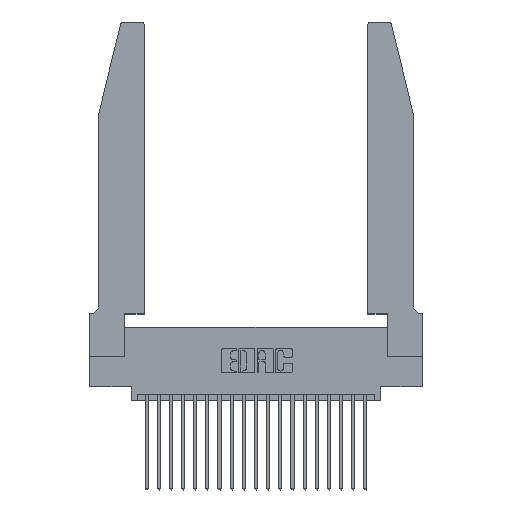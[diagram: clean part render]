
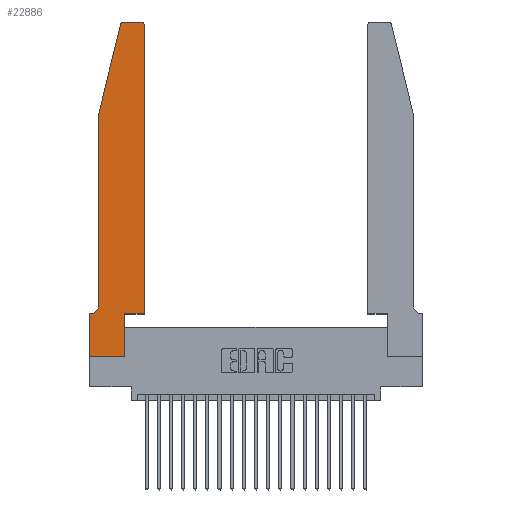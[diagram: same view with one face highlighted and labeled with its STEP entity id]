
A CAD part, top view. The second image highlights one B-rep face of the part: STEP entity #22886.
In plain terms, the highlighted planar face has unit normal (0, 0, 1).
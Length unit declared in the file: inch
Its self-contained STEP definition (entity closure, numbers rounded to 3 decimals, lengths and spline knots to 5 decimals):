
#38 = CIRCLE ( 'NONE', #16326, 0.07 ) ;
#225 = DIRECTION ( 'NONE',  ( 0., -1., 0. ) ) ;
#244 = VERTEX_POINT ( 'NONE', #14254 ) ;
#664 = VECTOR ( 'NONE', #12266, 39.37008 ) ;
#784 = DIRECTION ( 'NONE',  ( -1., 0., 0. ) ) ;
#834 = ORIENTED_EDGE ( 'NONE', *, *, #2104, .T. ) ;
#944 = ORIENTED_EDGE ( 'NONE', *, *, #11336, .T. ) ;
#1945 = ORIENTED_EDGE ( 'NONE', *, *, #15165, .T. ) ;
#2104 = EDGE_CURVE ( 'NONE', #244, #15278, #16944, .T. ) ;
#2153 = DIRECTION ( 'NONE',  ( 0., 0., 1. ) ) ;
#2366 = VERTEX_POINT ( 'NONE', #15646 ) ;
#2479 = EDGE_CURVE ( 'NONE', #20971, #8967, #14375, .T. ) ;
#3128 = AXIS2_PLACEMENT_3D ( 'NONE', #17118, #6433, #18855 ) ;
#3264 = DIRECTION ( 'NONE',  ( 1., 0., 0. ) ) ;
#3488 = DIRECTION ( 'NONE',  ( -1., 0., 0. ) ) ;
#3572 = ORIENTED_EDGE ( 'NONE', *, *, #12451, .T. ) ;
#3881 = PLANE ( 'NONE',  #18266 ) ;
#4040 = LINE ( 'NONE', #9130, #7724 ) ;
#4119 = VERTEX_POINT ( 'NONE', #5411 ) ;
#4292 = VECTOR ( 'NONE', #3488, 39.37008 ) ;
#4892 = DIRECTION ( 'NONE',  ( 0., 0., 1. ) ) ;
#4905 = LINE ( 'NONE', #13172, #14984 ) ;
#5411 = CARTESIAN_POINT ( 'NONE',  ( 0.0755, 2., 0.37 ) ) ;
#5440 = LINE ( 'NONE', #19428, #4292 ) ;
#6240 = CARTESIAN_POINT ( 'NONE',  ( 0.4505, 0.35, 0.37 ) ) ;
#6275 = FACE_OUTER_BOUND ( 'NONE', #11863, .T. ) ;
#6433 = DIRECTION ( 'NONE',  ( 0., 0., 1. ) ) ;
#6575 = ORIENTED_EDGE ( 'NONE', *, *, #20298, .T. ) ;
#6600 = VECTOR ( 'NONE', #225, 39.37008 ) ;
#6689 = ORIENTED_EDGE ( 'NONE', *, *, #2479, .T. ) ;
#7184 = VECTOR ( 'NONE', #18664, 39.37008 ) ;
#7588 = CARTESIAN_POINT ( 'NONE',  ( 0.4205, 2.75, 0.37 ) ) ;
#7648 = LINE ( 'NONE', #18235, #16572 ) ;
#7724 = VECTOR ( 'NONE', #10895, 39.37008 ) ;
#7786 = ORIENTED_EDGE ( 'NONE', *, *, #22735, .T. ) ;
#8215 = DIRECTION ( 'NONE',  ( 1., 0., 0. ) ) ;
#8338 = EDGE_CURVE ( 'NONE', #15278, #4119, #4905, .T. ) ;
#8515 = VERTEX_POINT ( 'NONE', #13626 ) ;
#8572 = DIRECTION ( 'NONE',  ( -1., 0., 0. ) ) ;
#8676 = VERTEX_POINT ( 'NONE', #14002 ) ;
#8967 = VERTEX_POINT ( 'NONE', #20052 ) ;
#9130 = CARTESIAN_POINT ( 'NONE',  ( 0., 0., 0.37 ) ) ;
#9265 = CARTESIAN_POINT ( 'NONE',  ( 0.0755, 2., 0.37 ) ) ;
#9797 = EDGE_CURVE ( 'NONE', #2366, #11171, #12679, .T. ) ;
#10109 = ORIENTED_EDGE ( 'NONE', *, *, #19187, .T. ) ;
#10895 = DIRECTION ( 'NONE',  ( 0., -1., 0. ) ) ;
#11171 = VERTEX_POINT ( 'NONE', #19843 ) ;
#11294 = CARTESIAN_POINT ( 'NONE',  ( 0.25487, 2.72718, 0.37 ) ) ;
#11336 = EDGE_CURVE ( 'NONE', #8676, #2366, #38, .T. ) ;
#11469 = LINE ( 'NONE', #17097, #19752 ) ;
#11509 = DIRECTION ( 'NONE',  ( 0., 0., -1. ) ) ;
#11863 = EDGE_LOOP ( 'NONE', ( #7786, #834, #14207, #10109, #944, #12807, #6575, #6689, #1945, #3572, #15208, #16627 ) ) ;
#11892 = LINE ( 'NONE', #9265, #6600 ) ;
#12108 = VECTOR ( 'NONE', #8572, 39.37008 ) ;
#12266 = DIRECTION ( 'NONE',  ( 1., 0., 0. ) ) ;
#12451 = EDGE_CURVE ( 'NONE', #8515, #19737, #11469, .T. ) ;
#12610 = CARTESIAN_POINT ( 'NONE',  ( 0., 0., 0.37 ) ) ;
#12679 = LINE ( 'NONE', #20879, #12108 ) ;
#12807 = ORIENTED_EDGE ( 'NONE', *, *, #9797, .T. ) ;
#12956 = CARTESIAN_POINT ( 'NONE',  ( 0.4505, 2.72, 0.37 ) ) ;
#13172 = CARTESIAN_POINT ( 'NONE',  ( 0.0755, 2., 0.37 ) ) ;
#13176 = AXIS2_PLACEMENT_3D ( 'NONE', #15329, #4892, #3264 ) ;
#13526 = CIRCLE ( 'NONE', #3128, 0.03 ) ;
#13626 = CARTESIAN_POINT ( 'NONE',  ( 0.2865, 0.35, 0.37 ) ) ;
#14002 = CARTESIAN_POINT ( 'NONE',  ( 0.0755, 0.42, 0.37 ) ) ;
#14207 = ORIENTED_EDGE ( 'NONE', *, *, #8338, .T. ) ;
#14254 = CARTESIAN_POINT ( 'NONE',  ( 0.284, 2.75, 0.37 ) ) ;
#14375 = LINE ( 'NONE', #12610, #664 ) ;
#14668 = DIRECTION ( 'NONE',  ( 1., 0., 0. ) ) ;
#14984 = VECTOR ( 'NONE', #18535, 39.37008 ) ;
#15165 = EDGE_CURVE ( 'NONE', #8967, #8515, #7648, .T. ) ;
#15208 = ORIENTED_EDGE ( 'NONE', *, *, #19898, .T. ) ;
#15278 = VERTEX_POINT ( 'NONE', #11294 ) ;
#15329 = CARTESIAN_POINT ( 'NONE',  ( 0.284, 2.72, 0.37 ) ) ;
#15646 = CARTESIAN_POINT ( 'NONE',  ( 0.0055, 0.35, 0.37 ) ) ;
#16326 = AXIS2_PLACEMENT_3D ( 'NONE', #22017, #11509, #784 ) ;
#16572 = VECTOR ( 'NONE', #18158, 39.37008 ) ;
#16627 = ORIENTED_EDGE ( 'NONE', *, *, #22505, .T. ) ;
#16944 = CIRCLE ( 'NONE', #13176, 0.03 ) ;
#17097 = CARTESIAN_POINT ( 'NONE',  ( 0.4505, 0.35, 0.37 ) ) ;
#17118 = CARTESIAN_POINT ( 'NONE',  ( 0.4205, 2.72, 0.37 ) ) ;
#18158 = DIRECTION ( 'NONE',  ( 0., 1., 0. ) ) ;
#18163 = CARTESIAN_POINT ( 'NONE',  ( 0.4505, 0.35, 0.37 ) ) ;
#18235 = CARTESIAN_POINT ( 'NONE',  ( 0.2865, 0.35, 0.37 ) ) ;
#18266 = AXIS2_PLACEMENT_3D ( 'NONE', #21595, #2153, #14668 ) ;
#18535 = DIRECTION ( 'NONE',  ( -0.239, -0.971, 0. ) ) ;
#18664 = DIRECTION ( 'NONE',  ( 0., 1., 0. ) ) ;
#18855 = DIRECTION ( 'NONE',  ( 1., 0., 0. ) ) ;
#19187 = EDGE_CURVE ( 'NONE', #4119, #8676, #11892, .T. ) ;
#19428 = CARTESIAN_POINT ( 'NONE',  ( 0.2605, 2.75, 0.37 ) ) ;
#19732 = VERTEX_POINT ( 'NONE', #12956 ) ;
#19737 = VERTEX_POINT ( 'NONE', #18163 ) ;
#19752 = VECTOR ( 'NONE', #8215, 39.37008 ) ;
#19843 = CARTESIAN_POINT ( 'NONE',  ( 0., 0.35, 0.37 ) ) ;
#19898 = EDGE_CURVE ( 'NONE', #19737, #19732, #20691, .T. ) ;
#20052 = CARTESIAN_POINT ( 'NONE',  ( 0.2865, 0., 0.37 ) ) ;
#20298 = EDGE_CURVE ( 'NONE', #11171, #20971, #4040, .T. ) ;
#20691 = LINE ( 'NONE', #6240, #7184 ) ;
#20854 = CARTESIAN_POINT ( 'NONE',  ( 0., 0., 0.37 ) ) ;
#20879 = CARTESIAN_POINT ( 'NONE',  ( 0.0755, 0.35, 0.37 ) ) ;
#20971 = VERTEX_POINT ( 'NONE', #20854 ) ;
#21595 = CARTESIAN_POINT ( 'NONE',  ( 0., 0.35, 0.37 ) ) ;
#21806 = VERTEX_POINT ( 'NONE', #7588 ) ;
#22017 = CARTESIAN_POINT ( 'NONE',  ( 0.0055, 0.42, 0.37 ) ) ;
#22505 = EDGE_CURVE ( 'NONE', #19732, #21806, #13526, .T. ) ;
#22735 = EDGE_CURVE ( 'NONE', #21806, #244, #5440, .T. ) ;
#22886 = ADVANCED_FACE ( 'NONE', ( #6275 ), #3881, .T. ) ;
